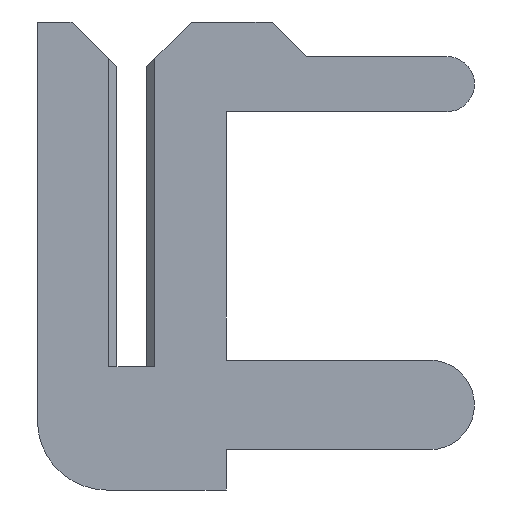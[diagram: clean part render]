
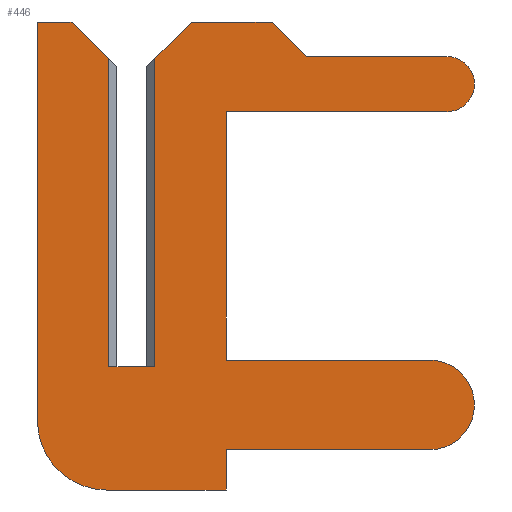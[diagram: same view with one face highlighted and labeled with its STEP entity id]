
A CAD part, left-side view. The second image highlights one B-rep face of the part: STEP entity #446.
In plain terms, the highlighted planar face has unit normal (-1, 0, 0).
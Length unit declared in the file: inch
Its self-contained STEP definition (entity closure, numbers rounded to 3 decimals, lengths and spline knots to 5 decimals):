
#6 = EDGE_CURVE ( 'NONE', #284, #119, #783, .T. ) ;
#9 = DIRECTION ( 'NONE',  ( 0., 0., 1. ) ) ;
#20 = DIRECTION ( 'NONE',  ( 0., -1., 0. ) ) ;
#39 = VECTOR ( 'NONE', #931, 39.37008 ) ;
#45 = CARTESIAN_POINT ( 'NONE',  ( -0.01, -0.1295, -0.0165 ) ) ;
#52 = LINE ( 'NONE', #717, #1087 ) ;
#56 = DIRECTION ( 'NONE',  ( 0., -1., 0. ) ) ;
#64 = VECTOR ( 'NONE', #219, 39.37008 ) ;
#75 = EDGE_CURVE ( 'NONE', #537, #395, #569, .T. ) ;
#82 = CARTESIAN_POINT ( 'NONE',  ( -0.01, -0.041, -0.036 ) ) ;
#84 = LINE ( 'NONE', #397, #681 ) ;
#87 = LINE ( 'NONE', #345, #729 ) ;
#90 = VERTEX_POINT ( 'NONE', #591 ) ;
#94 = VECTOR ( 'NONE', #579, 39.37008 ) ;
#103 = VERTEX_POINT ( 'NONE', #1079 ) ;
#110 = AXIS2_PLACEMENT_3D ( 'NONE', #1160, #1061, #763 ) ;
#117 = FACE_OUTER_BOUND ( 'NONE', #209, .T. ) ;
#119 = VERTEX_POINT ( 'NONE', #374 ) ;
#143 = VERTEX_POINT ( 'NONE', #495 ) ;
#149 = ORIENTED_EDGE ( 'NONE', *, *, #885, .F. ) ;
#159 = VERTEX_POINT ( 'NONE', #891 ) ;
#160 = DIRECTION ( 'NONE',  ( 0., 0., 1. ) ) ;
#165 = CARTESIAN_POINT ( 'NONE',  ( -0.01, 0.026, 0.15 ) ) ;
#205 = CARTESIAN_POINT ( 'NONE',  ( -0.01, 0.041, -0.0235 ) ) ;
#209 = EDGE_LOOP ( 'NONE', ( #755, #1129, #333, #1260, #1271, #149, #977, #1075, #511, #338, #1212, #657, #948, #914, #674, #1013, #346, #979, #224 ) ) ;
#210 = CARTESIAN_POINT ( 'NONE',  ( -0.01, -0.01, 0.134 ) ) ;
#215 = CARTESIAN_POINT ( 'NONE',  ( -0.01, 0.01, 0.134 ) ) ;
#219 = DIRECTION ( 'NONE',  ( 0., 0., -1. ) ) ;
#220 = LINE ( 'NONE', #417, #1182 ) ;
#222 = CARTESIAN_POINT ( 'NONE',  ( -0.01, 0.011, -0.0535 ) ) ;
#224 = ORIENTED_EDGE ( 'NONE', *, *, #602, .F. ) ;
#228 = CARTESIAN_POINT ( 'NONE',  ( -0.01, -0.1295, -0.036 ) ) ;
#261 = EDGE_CURVE ( 'NONE', #411, #1094, #52, .T. ) ;
#271 = CIRCLE ( 'NONE', #110, 0.03 ) ;
#279 = DIRECTION ( 'NONE',  ( 0., 1., 0. ) ) ;
#284 = VERTEX_POINT ( 'NONE', #228 ) ;
#286 = EDGE_CURVE ( 'NONE', #635, #159, #1124, .T. ) ;
#289 = VECTOR ( 'NONE', #279, 39.37008 ) ;
#294 = CARTESIAN_POINT ( 'NONE',  ( -0.01, 0.041, 0.15 ) ) ;
#295 = CARTESIAN_POINT ( 'NONE',  ( -0.01, -0.1295, 0.003 ) ) ;
#298 = CARTESIAN_POINT ( 'NONE',  ( -0.01, -0.137, 0.135 ) ) ;
#323 = EDGE_CURVE ( 'NONE', #411, #143, #1057, .T. ) ;
#333 = ORIENTED_EDGE ( 'NONE', *, *, #323, .F. ) ;
#338 = ORIENTED_EDGE ( 'NONE', *, *, #1119, .F. ) ;
#345 = CARTESIAN_POINT ( 'NONE',  ( -0.01, -0.041, 0.003 ) ) ;
#346 = ORIENTED_EDGE ( 'NONE', *, *, #423, .F. ) ;
#364 = EDGE_CURVE ( 'NONE', #1264, #445, #443, .T. ) ;
#374 = CARTESIAN_POINT ( 'NONE',  ( -0.01, -0.041, -0.036 ) ) ;
#383 = CARTESIAN_POINT ( 'NONE',  ( -0.01, 0.026, 0.15 ) ) ;
#384 = EDGE_CURVE ( 'NONE', #923, #143, #84, .T. ) ;
#392 = EDGE_CURVE ( 'NONE', #923, #90, #683, .T. ) ;
#395 = VERTEX_POINT ( 'NONE', #973 ) ;
#397 = CARTESIAN_POINT ( 'NONE',  ( -0.01, -0.01, 0.15 ) ) ;
#411 = VERTEX_POINT ( 'NONE', #659 ) ;
#416 = CARTESIAN_POINT ( 'NONE',  ( -0.01, -0.041, -0.0535 ) ) ;
#417 = CARTESIAN_POINT ( 'NONE',  ( -0.01, -0.1295, 0.003 ) ) ;
#423 = EDGE_CURVE ( 'NONE', #159, #103, #1033, .T. ) ;
#440 = CIRCLE ( 'NONE', #738, 0.0195 ) ;
#443 = LINE ( 'NONE', #294, #39 ) ;
#445 = VERTEX_POINT ( 'NONE', #818 ) ;
#446 = ADVANCED_FACE ( 'NONE', ( #117 ), #1114, .T. ) ;
#461 = DIRECTION ( 'NONE',  ( 1., 0., 0. ) ) ;
#474 = EDGE_CURVE ( 'NONE', #488, #1017, #220, .T. ) ;
#485 = LINE ( 'NONE', #222, #1084 ) ;
#488 = VERTEX_POINT ( 'NONE', #901 ) ;
#495 = CARTESIAN_POINT ( 'NONE',  ( -0.01, -0.01, 0. ) ) ;
#508 = VECTOR ( 'NONE', #988, 39.37008 ) ;
#511 = ORIENTED_EDGE ( 'NONE', *, *, #1256, .F. ) ;
#515 = DIRECTION ( 'NONE',  ( 0., -0.707, -0.707 ) ) ;
#529 = DIRECTION ( 'NONE',  ( 0., -0.707, -0.707 ) ) ;
#532 = VECTOR ( 'NONE', #515, 39.37008 ) ;
#537 = VERTEX_POINT ( 'NONE', #911 ) ;
#543 = CARTESIAN_POINT ( 'NONE',  ( -0.01, -0.061, 0.15 ) ) ;
#569 = LINE ( 'NONE', #779, #289 ) ;
#579 = DIRECTION ( 'NONE',  ( 0., -0.707, 0.707 ) ) ;
#591 = CARTESIAN_POINT ( 'NONE',  ( -0.01, -0.026, 0.15 ) ) ;
#592 = LINE ( 'NONE', #688, #532 ) ;
#599 = DIRECTION ( 'NONE',  ( 0., -1., 0. ) ) ;
#602 = EDGE_CURVE ( 'NONE', #90, #635, #987, .T. ) ;
#612 = VECTOR ( 'NONE', #1045, 39.37008 ) ;
#616 = EDGE_CURVE ( 'NONE', #1222, #1264, #271, .T. ) ;
#635 = VERTEX_POINT ( 'NONE', #543 ) ;
#648 = VECTOR ( 'NONE', #56, 39.37008 ) ;
#649 = CARTESIAN_POINT ( 'NONE',  ( -0.01, -0.076, 0.135 ) ) ;
#657 = ORIENTED_EDGE ( 'NONE', *, *, #767, .F. ) ;
#659 = CARTESIAN_POINT ( 'NONE',  ( -0.01, 0.01, 0. ) ) ;
#674 = ORIENTED_EDGE ( 'NONE', *, *, #75, .F. ) ;
#681 = VECTOR ( 'NONE', #998, 39.37008 ) ;
#683 = LINE ( 'NONE', #894, #94 ) ;
#685 = CARTESIAN_POINT ( 'NONE',  ( -0.01, -0.137, 0.123 ) ) ;
#688 = CARTESIAN_POINT ( 'NONE',  ( -0.01, 0.0065, 0.1305 ) ) ;
#700 = AXIS2_PLACEMENT_3D ( 'NONE', #685, #770, #160 ) ;
#716 = DIRECTION ( 'NONE',  ( -1., 0., 0. ) ) ;
#717 = CARTESIAN_POINT ( 'NONE',  ( -0.01, 0.01, -0.0235 ) ) ;
#729 = VECTOR ( 'NONE', #1272, 39.37008 ) ;
#738 = AXIS2_PLACEMENT_3D ( 'NONE', #45, #461, #1262 ) ;
#748 = VERTEX_POINT ( 'NONE', #1247 ) ;
#755 = ORIENTED_EDGE ( 'NONE', *, *, #392, .F. ) ;
#761 = VECTOR ( 'NONE', #599, 39.37008 ) ;
#763 = DIRECTION ( 'NONE',  ( 0., 0., 1. ) ) ;
#767 = EDGE_CURVE ( 'NONE', #1017, #284, #440, .T. ) ;
#770 = DIRECTION ( 'NONE',  ( 1., 0., 0. ) ) ;
#779 = CARTESIAN_POINT ( 'NONE',  ( -0.01, -0.041, 0.111 ) ) ;
#783 = LINE ( 'NONE', #82, #508 ) ;
#818 = CARTESIAN_POINT ( 'NONE',  ( -0.01, 0.041, 0.15 ) ) ;
#824 = DIRECTION ( 'NONE',  ( 0., 0., 1. ) ) ;
#825 = EDGE_CURVE ( 'NONE', #395, #488, #87, .T. ) ;
#836 = CARTESIAN_POINT ( 'NONE',  ( -0.01, 0.0065, 0. ) ) ;
#852 = LINE ( 'NONE', #416, #64 ) ;
#885 = EDGE_CURVE ( 'NONE', #445, #1062, #943, .T. ) ;
#891 = CARTESIAN_POINT ( 'NONE',  ( -0.01, -0.076, 0.135 ) ) ;
#894 = CARTESIAN_POINT ( 'NONE',  ( -0.01, -0.0065, 0.1305 ) ) ;
#901 = CARTESIAN_POINT ( 'NONE',  ( -0.01, -0.041, 0.003 ) ) ;
#909 = EDGE_CURVE ( 'NONE', #103, #537, #1191, .T. ) ;
#911 = CARTESIAN_POINT ( 'NONE',  ( -0.01, -0.137, 0.111 ) ) ;
#914 = ORIENTED_EDGE ( 'NONE', *, *, #825, .F. ) ;
#917 = CARTESIAN_POINT ( 'NONE',  ( -0.01, 0.011, -0.0235 ) ) ;
#923 = VERTEX_POINT ( 'NONE', #210 ) ;
#931 = DIRECTION ( 'NONE',  ( 0., 0., 1. ) ) ;
#943 = LINE ( 'NONE', #165, #1139 ) ;
#948 = ORIENTED_EDGE ( 'NONE', *, *, #474, .F. ) ;
#950 = CARTESIAN_POINT ( 'NONE',  ( -0.01, -0.026, 0.15 ) ) ;
#955 = AXIS2_PLACEMENT_3D ( 'NONE', #917, #716, #9 ) ;
#973 = CARTESIAN_POINT ( 'NONE',  ( -0.01, -0.041, 0.111 ) ) ;
#977 = ORIENTED_EDGE ( 'NONE', *, *, #364, .F. ) ;
#979 = ORIENTED_EDGE ( 'NONE', *, *, #286, .F. ) ;
#987 = LINE ( 'NONE', #950, #648 ) ;
#988 = DIRECTION ( 'NONE',  ( 0., 1., 0. ) ) ;
#998 = DIRECTION ( 'NONE',  ( 0., 0., -1. ) ) ;
#1013 = ORIENTED_EDGE ( 'NONE', *, *, #909, .F. ) ;
#1017 = VERTEX_POINT ( 'NONE', #295 ) ;
#1018 = CARTESIAN_POINT ( 'NONE',  ( -0.01, 0.011, -0.0535 ) ) ;
#1033 = LINE ( 'NONE', #298, #761 ) ;
#1045 = DIRECTION ( 'NONE',  ( 0., -1., 0. ) ) ;
#1057 = LINE ( 'NONE', #836, #612 ) ;
#1061 = DIRECTION ( 'NONE',  ( 1., 0., 0. ) ) ;
#1062 = VERTEX_POINT ( 'NONE', #383 ) ;
#1075 = ORIENTED_EDGE ( 'NONE', *, *, #616, .F. ) ;
#1079 = CARTESIAN_POINT ( 'NONE',  ( -0.01, -0.137, 0.135 ) ) ;
#1084 = VECTOR ( 'NONE', #1228, 39.37008 ) ;
#1087 = VECTOR ( 'NONE', #824, 39.37008 ) ;
#1089 = EDGE_CURVE ( 'NONE', #1062, #1094, #592, .T. ) ;
#1094 = VERTEX_POINT ( 'NONE', #215 ) ;
#1114 = PLANE ( 'NONE',  #955 ) ;
#1119 = EDGE_CURVE ( 'NONE', #119, #748, #852, .T. ) ;
#1124 = LINE ( 'NONE', #649, #1210 ) ;
#1129 = ORIENTED_EDGE ( 'NONE', *, *, #384, .T. ) ;
#1139 = VECTOR ( 'NONE', #1282, 39.37008 ) ;
#1160 = CARTESIAN_POINT ( 'NONE',  ( -0.01, 0.011, -0.0235 ) ) ;
#1182 = VECTOR ( 'NONE', #20, 39.37008 ) ;
#1191 = CIRCLE ( 'NONE', #700, 0.012 ) ;
#1210 = VECTOR ( 'NONE', #529, 39.37008 ) ;
#1212 = ORIENTED_EDGE ( 'NONE', *, *, #6, .F. ) ;
#1222 = VERTEX_POINT ( 'NONE', #1018 ) ;
#1228 = DIRECTION ( 'NONE',  ( 0., 1., 0. ) ) ;
#1247 = CARTESIAN_POINT ( 'NONE',  ( -0.01, -0.041, -0.0535 ) ) ;
#1256 = EDGE_CURVE ( 'NONE', #748, #1222, #485, .T. ) ;
#1260 = ORIENTED_EDGE ( 'NONE', *, *, #261, .T. ) ;
#1262 = DIRECTION ( 'NONE',  ( 0., 0., 1. ) ) ;
#1264 = VERTEX_POINT ( 'NONE', #205 ) ;
#1271 = ORIENTED_EDGE ( 'NONE', *, *, #1089, .F. ) ;
#1272 = DIRECTION ( 'NONE',  ( 0., 0., -1. ) ) ;
#1282 = DIRECTION ( 'NONE',  ( 0., -1., 0. ) ) ;
